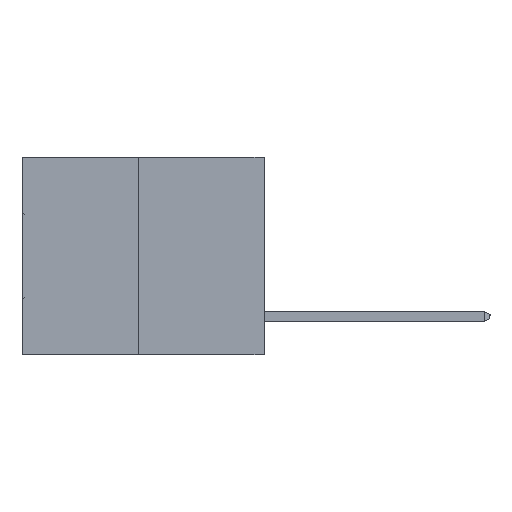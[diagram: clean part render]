
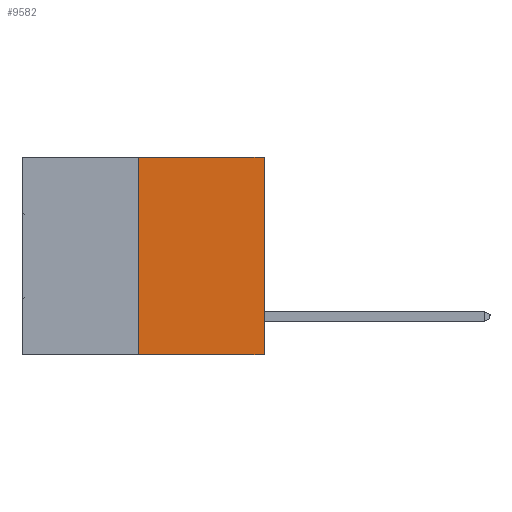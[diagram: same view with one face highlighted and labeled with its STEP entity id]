
A CAD part, left-side view. The second image highlights one B-rep face of the part: STEP entity #9582.
In plain terms, the highlighted planar face has unit normal (-1, 0, 0).
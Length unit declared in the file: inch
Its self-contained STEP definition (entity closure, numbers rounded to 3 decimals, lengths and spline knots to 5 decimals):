
#42 = LINE ( 'NONE', #34749, #6116 ) ;
#2533 = VERTEX_POINT ( 'NONE', #7709 ) ;
#3809 = ORIENTED_EDGE ( 'NONE', *, *, #34806, .T. ) ;
#4368 = DIRECTION ( 'NONE',  ( 0., 0., 1. ) ) ;
#4643 = CARTESIAN_POINT ( 'NONE',  ( 0., 0.6, 0. ) ) ;
#6116 = VECTOR ( 'NONE', #29121, 39.37008 ) ;
#7593 = DIRECTION ( 'NONE',  ( 0., 0., -1. ) ) ;
#7709 = CARTESIAN_POINT ( 'NONE',  ( 0., 0., -0.49 ) ) ;
#8484 = LINE ( 'NONE', #4643, #20233 ) ;
#9582 = ADVANCED_FACE ( 'NONE', ( #18091 ), #24218, .F. ) ;
#10626 = VERTEX_POINT ( 'NONE', #11263 ) ;
#11263 = CARTESIAN_POINT ( 'NONE',  ( 0., 0.312, 0. ) ) ;
#11516 = ORIENTED_EDGE ( 'NONE', *, *, #11968, .F. ) ;
#11968 = EDGE_CURVE ( 'NONE', #10626, #34218, #8484, .T. ) ;
#12953 = CARTESIAN_POINT ( 'NONE',  ( 0., 0., 0. ) ) ;
#14124 = LINE ( 'NONE', #12953, #22349 ) ;
#14374 = EDGE_CURVE ( 'NONE', #26934, #2533, #42, .T. ) ;
#15625 = EDGE_LOOP ( 'NONE', ( #21253, #31276, #3809, #11516 ) ) ;
#18091 = FACE_OUTER_BOUND ( 'NONE', #15625, .T. ) ;
#19765 = VECTOR ( 'NONE', #22732, 39.37008 ) ;
#19961 = CARTESIAN_POINT ( 'NONE',  ( 0., 0.312, -0.49 ) ) ;
#20233 = VECTOR ( 'NONE', #21508, 39.37008 ) ;
#21106 = DIRECTION ( 'NONE',  ( 1., 0., 0. ) ) ;
#21253 = ORIENTED_EDGE ( 'NONE', *, *, #29094, .F. ) ;
#21508 = DIRECTION ( 'NONE',  ( 0., -1., 0. ) ) ;
#22349 = VECTOR ( 'NONE', #4368, 39.37008 ) ;
#22732 = DIRECTION ( 'NONE',  ( 0., 0., 1. ) ) ;
#23058 = CARTESIAN_POINT ( 'NONE',  ( 0., 0., 0. ) ) ;
#24218 = PLANE ( 'NONE',  #35366 ) ;
#26041 = CARTESIAN_POINT ( 'NONE',  ( 0., 0.312, -0.49 ) ) ;
#26886 = CARTESIAN_POINT ( 'NONE',  ( 0., 0.6, 0. ) ) ;
#26934 = VERTEX_POINT ( 'NONE', #26041 ) ;
#27981 = LINE ( 'NONE', #19961, #19765 ) ;
#29094 = EDGE_CURVE ( 'NONE', #26934, #10626, #27981, .T. ) ;
#29121 = DIRECTION ( 'NONE',  ( 0., -1., 0. ) ) ;
#31276 = ORIENTED_EDGE ( 'NONE', *, *, #14374, .T. ) ;
#34218 = VERTEX_POINT ( 'NONE', #23058 ) ;
#34749 = CARTESIAN_POINT ( 'NONE',  ( 0., 0.6, -0.49 ) ) ;
#34806 = EDGE_CURVE ( 'NONE', #2533, #34218, #14124, .T. ) ;
#35366 = AXIS2_PLACEMENT_3D ( 'NONE', #26886, #21106, #7593 ) ;
